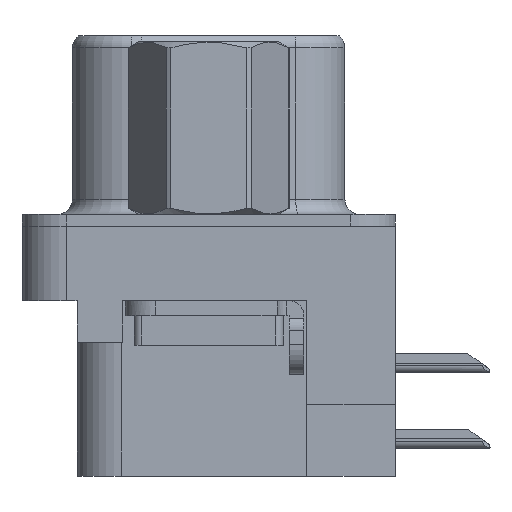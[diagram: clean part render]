
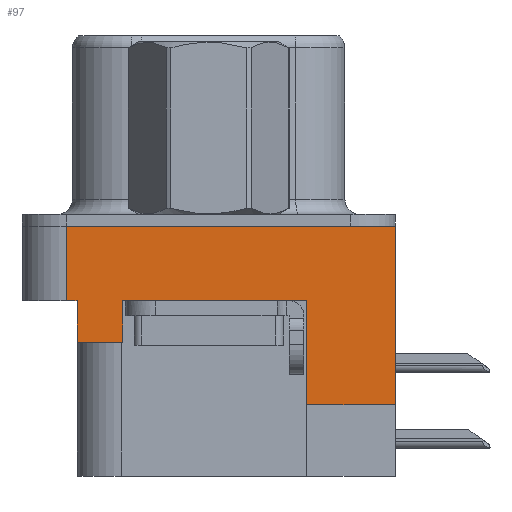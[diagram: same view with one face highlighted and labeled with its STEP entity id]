
A CAD part, left-side view. The second image highlights one B-rep face of the part: STEP entity #97.
In plain terms, the highlighted planar face has unit normal (-1, 0, 0).
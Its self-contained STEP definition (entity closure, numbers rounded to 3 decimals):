
#97 = ADVANCED_FACE ( 'NONE', ( #19200 ), #652, .T. ) ;
#225 = EDGE_CURVE ( 'NONE', #12017, #17213, #26324, .T. ) ;
#652 = PLANE ( 'NONE',  #14594 ) ;
#1034 = VERTEX_POINT ( 'NONE', #25863 ) ;
#1156 = EDGE_CURVE ( 'NONE', #1034, #22760, #25964, .T. ) ;
#1245 = ORIENTED_EDGE ( 'NONE', *, *, #1156, .F. ) ;
#1301 = EDGE_CURVE ( 'NONE', #17011, #12017, #13608, .T. ) ;
#1351 = VERTEX_POINT ( 'NONE', #6426 ) ;
#2154 = CARTESIAN_POINT ( 'NONE',  ( -3., 2.895, -2.5 ) ) ;
#2758 = VECTOR ( 'NONE', #23705, 1000. ) ;
#3219 = DIRECTION ( 'NONE',  ( 0., -1., 0. ) ) ;
#3862 = VECTOR ( 'NONE', #18257, 1000. ) ;
#4218 = CARTESIAN_POINT ( 'NONE',  ( -3., -3.295, -2.5 ) ) ;
#4327 = ORIENTED_EDGE ( 'NONE', *, *, #23086, .F. ) ;
#4700 = VERTEX_POINT ( 'NONE', #22988 ) ;
#5146 = LINE ( 'NONE', #13768, #15547 ) ;
#5619 = VECTOR ( 'NONE', #21130, 1000. ) ;
#5922 = DIRECTION ( 'NONE',  ( 0., 0., 1. ) ) ;
#5978 = EDGE_CURVE ( 'NONE', #6154, #1351, #5146, .T. ) ;
#6154 = VERTEX_POINT ( 'NONE', #10594 ) ;
#6272 = CARTESIAN_POINT ( 'NONE',  ( -3., 4.775, -2.5 ) ) ;
#6426 = CARTESIAN_POINT ( 'NONE',  ( -3., -3.295, -6. ) ) ;
#6782 = CARTESIAN_POINT ( 'NONE',  ( -3., -6.275, 0. ) ) ;
#7057 = ORIENTED_EDGE ( 'NONE', *, *, #22547, .F. ) ;
#7095 = CARTESIAN_POINT ( 'NONE',  ( -3., -6.275, -2.5 ) ) ;
#7993 = EDGE_CURVE ( 'NONE', #19334, #4700, #10308, .T. ) ;
#8061 = CARTESIAN_POINT ( 'NONE',  ( -3., -6.275, 0. ) ) ;
#8867 = DIRECTION ( 'NONE',  ( 0., -1., 0. ) ) ;
#9042 = LINE ( 'NONE', #6782, #24943 ) ;
#9604 = LINE ( 'NONE', #13338, #2758 ) ;
#9758 = VECTOR ( 'NONE', #3219, 1000. ) ;
#10308 = LINE ( 'NONE', #19664, #20723 ) ;
#10323 = DIRECTION ( 'NONE',  ( 0., 0., 1. ) ) ;
#10569 = DIRECTION ( 'NONE',  ( 0., 0., 1. ) ) ;
#10594 = CARTESIAN_POINT ( 'NONE',  ( -3., -6.275, -6. ) ) ;
#11157 = LINE ( 'NONE', #14834, #5619 ) ;
#11237 = ORIENTED_EDGE ( 'NONE', *, *, #19239, .T. ) ;
#11781 = DIRECTION ( 'NONE',  ( 0., 1., 0. ) ) ;
#12017 = VERTEX_POINT ( 'NONE', #2154 ) ;
#12698 = EDGE_LOOP ( 'NONE', ( #16664, #11237, #20665, #24948, #19744, #1245, #4327, #22471, #19939, #7057 ) ) ;
#13338 = CARTESIAN_POINT ( 'NONE',  ( -3., 4.425, -3.9 ) ) ;
#13550 = LINE ( 'NONE', #20476, #24601 ) ;
#13608 = LINE ( 'NONE', #24945, #17205 ) ;
#13768 = CARTESIAN_POINT ( 'NONE',  ( -3., -6.495, -6. ) ) ;
#14594 = AXIS2_PLACEMENT_3D ( 'NONE', #7095, #23075, #26779 ) ;
#14834 = CARTESIAN_POINT ( 'NONE',  ( -3., -6.275, -2.5 ) ) ;
#15350 = VERTEX_POINT ( 'NONE', #8061 ) ;
#15547 = VECTOR ( 'NONE', #11781, 1000. ) ;
#16008 = VECTOR ( 'NONE', #10569, 1000. ) ;
#16664 = ORIENTED_EDGE ( 'NONE', *, *, #5978, .F. ) ;
#17011 = VERTEX_POINT ( 'NONE', #22407 ) ;
#17205 = VECTOR ( 'NONE', #10323, 1000. ) ;
#17213 = VERTEX_POINT ( 'NONE', #4218 ) ;
#18257 = DIRECTION ( 'NONE',  ( 0., 0., 1. ) ) ;
#18335 = CARTESIAN_POINT ( 'NONE',  ( -3., 4.425, -3.9 ) ) ;
#18548 = CARTESIAN_POINT ( 'NONE',  ( -3., 4.425, -2.5 ) ) ;
#18921 = EDGE_CURVE ( 'NONE', #4700, #15350, #9042, .T. ) ;
#19200 = FACE_OUTER_BOUND ( 'NONE', #12698, .T. ) ;
#19239 = EDGE_CURVE ( 'NONE', #6154, #15350, #13550, .T. ) ;
#19334 = VERTEX_POINT ( 'NONE', #6272 ) ;
#19664 = CARTESIAN_POINT ( 'NONE',  ( -3., 4.775, -2.5 ) ) ;
#19744 = ORIENTED_EDGE ( 'NONE', *, *, #21892, .T. ) ;
#19939 = ORIENTED_EDGE ( 'NONE', *, *, #225, .T. ) ;
#20476 = CARTESIAN_POINT ( 'NONE',  ( -3., -6.275, -2.5 ) ) ;
#20665 = ORIENTED_EDGE ( 'NONE', *, *, #18921, .F. ) ;
#20723 = VECTOR ( 'NONE', #21741, 1000. ) ;
#20953 = CARTESIAN_POINT ( 'NONE',  ( -3., -3.295, -8.4 ) ) ;
#21130 = DIRECTION ( 'NONE',  ( 0., -1., 0. ) ) ;
#21741 = DIRECTION ( 'NONE',  ( 0., 0., 1. ) ) ;
#21892 = EDGE_CURVE ( 'NONE', #19334, #22760, #11157, .T. ) ;
#22407 = CARTESIAN_POINT ( 'NONE',  ( -3., 2.895, -3.9 ) ) ;
#22471 = ORIENTED_EDGE ( 'NONE', *, *, #1301, .T. ) ;
#22547 = EDGE_CURVE ( 'NONE', #1351, #17213, #27002, .T. ) ;
#22760 = VERTEX_POINT ( 'NONE', #18548 ) ;
#22988 = CARTESIAN_POINT ( 'NONE',  ( -3., 4.775, 0. ) ) ;
#23075 = DIRECTION ( 'NONE',  ( -1., 0., 0. ) ) ;
#23086 = EDGE_CURVE ( 'NONE', #17011, #1034, #9604, .T. ) ;
#23705 = DIRECTION ( 'NONE',  ( 0., 1., 0. ) ) ;
#24601 = VECTOR ( 'NONE', #5922, 1000. ) ;
#24943 = VECTOR ( 'NONE', #8867, 1000. ) ;
#24945 = CARTESIAN_POINT ( 'NONE',  ( -3., 2.895, -3.9 ) ) ;
#24948 = ORIENTED_EDGE ( 'NONE', *, *, #7993, .F. ) ;
#25863 = CARTESIAN_POINT ( 'NONE',  ( -3., 4.425, -3.9 ) ) ;
#25964 = LINE ( 'NONE', #18335, #3862 ) ;
#26324 = LINE ( 'NONE', #26371, #9758 ) ;
#26371 = CARTESIAN_POINT ( 'NONE',  ( -3., -6.275, -2.5 ) ) ;
#26779 = DIRECTION ( 'NONE',  ( 0., 0., 1. ) ) ;
#27002 = LINE ( 'NONE', #20953, #16008 ) ;
